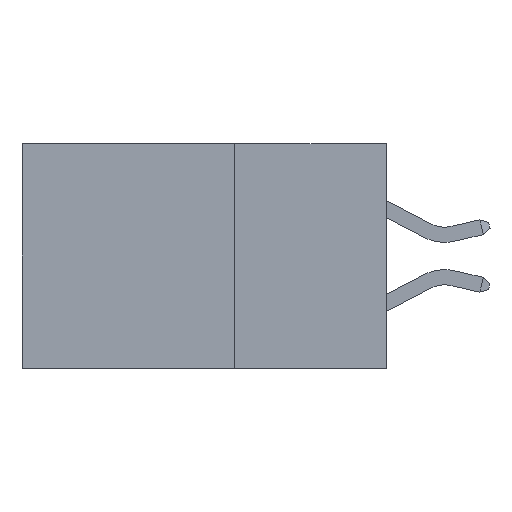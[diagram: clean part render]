
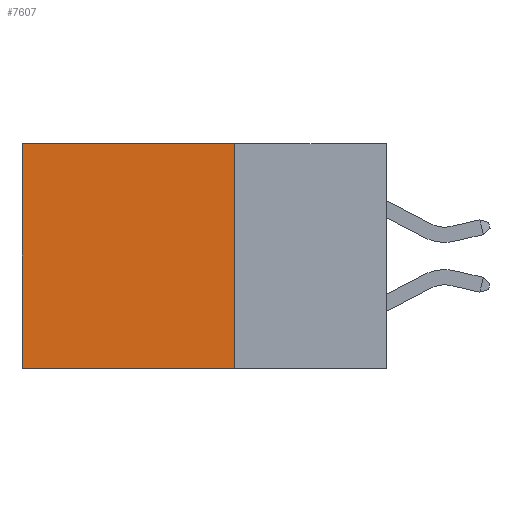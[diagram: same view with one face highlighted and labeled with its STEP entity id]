
A CAD part, left-side view. The second image highlights one B-rep face of the part: STEP entity #7607.
In plain terms, the highlighted planar face has unit normal (-1, 0, 0).
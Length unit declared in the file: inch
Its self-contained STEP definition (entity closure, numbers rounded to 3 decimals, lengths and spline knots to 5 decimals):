
#403 = FACE_OUTER_BOUND ( 'NONE', #2417, .T. ) ;
#584 = AXIS2_PLACEMENT_3D ( 'NONE', #8042, #4434, #6093 ) ;
#1522 = CARTESIAN_POINT ( 'NONE',  ( 0.298, 0.25, -0.37 ) ) ;
#1706 = VERTEX_POINT ( 'NONE', #9765 ) ;
#2095 = CARTESIAN_POINT ( 'NONE',  ( 0.298, 0.6, 0. ) ) ;
#2417 = EDGE_LOOP ( 'NONE', ( #17587, #11663, #6642, #21014 ) ) ;
#3456 = VERTEX_POINT ( 'NONE', #2095 ) ;
#3883 = CARTESIAN_POINT ( 'NONE',  ( 0.298, 0.25, 0. ) ) ;
#4230 = LINE ( 'NONE', #1522, #6213 ) ;
#4434 = DIRECTION ( 'NONE',  ( 1., 0., 0. ) ) ;
#5023 = CARTESIAN_POINT ( 'NONE',  ( 0.298, 0.6, 0. ) ) ;
#5223 = VERTEX_POINT ( 'NONE', #21277 ) ;
#5322 = LINE ( 'NONE', #5023, #22610 ) ;
#5347 = EDGE_CURVE ( 'NONE', #15313, #1706, #4230, .T. ) ;
#6093 = DIRECTION ( 'NONE',  ( 0., 0., -1. ) ) ;
#6213 = VECTOR ( 'NONE', #12413, 39.37008 ) ;
#6642 = ORIENTED_EDGE ( 'NONE', *, *, #18101, .F. ) ;
#7035 = CARTESIAN_POINT ( 'NONE',  ( 0.298, 0.25, 0. ) ) ;
#7607 = ADVANCED_FACE ( 'NONE', ( #403 ), #7874, .F. ) ;
#7874 = PLANE ( 'NONE',  #584 ) ;
#8042 = CARTESIAN_POINT ( 'NONE',  ( 0.298, 0.25, 0. ) ) ;
#9765 = CARTESIAN_POINT ( 'NONE',  ( 0.298, 0.6, -0.37 ) ) ;
#11663 = ORIENTED_EDGE ( 'NONE', *, *, #5347, .F. ) ;
#12413 = DIRECTION ( 'NONE',  ( 0., 1., 0. ) ) ;
#12662 = VECTOR ( 'NONE', #18825, 39.37008 ) ;
#15313 = VERTEX_POINT ( 'NONE', #17024 ) ;
#16397 = DIRECTION ( 'NONE',  ( 0., 0., -1. ) ) ;
#17024 = CARTESIAN_POINT ( 'NONE',  ( 0.298, 0.25, -0.37 ) ) ;
#17587 = ORIENTED_EDGE ( 'NONE', *, *, #21619, .T. ) ;
#17640 = VECTOR ( 'NONE', #16397, 39.37008 ) ;
#18101 = EDGE_CURVE ( 'NONE', #5223, #15313, #22799, .T. ) ;
#18825 = DIRECTION ( 'NONE',  ( 0., 1., 0. ) ) ;
#18944 = EDGE_CURVE ( 'NONE', #5223, #3456, #23330, .T. ) ;
#21014 = ORIENTED_EDGE ( 'NONE', *, *, #18944, .T. ) ;
#21277 = CARTESIAN_POINT ( 'NONE',  ( 0.298, 0.25, 0. ) ) ;
#21535 = DIRECTION ( 'NONE',  ( 0., 0., -1. ) ) ;
#21619 = EDGE_CURVE ( 'NONE', #3456, #1706, #5322, .T. ) ;
#22610 = VECTOR ( 'NONE', #21535, 39.37008 ) ;
#22799 = LINE ( 'NONE', #7035, #17640 ) ;
#23330 = LINE ( 'NONE', #3883, #12662 ) ;
